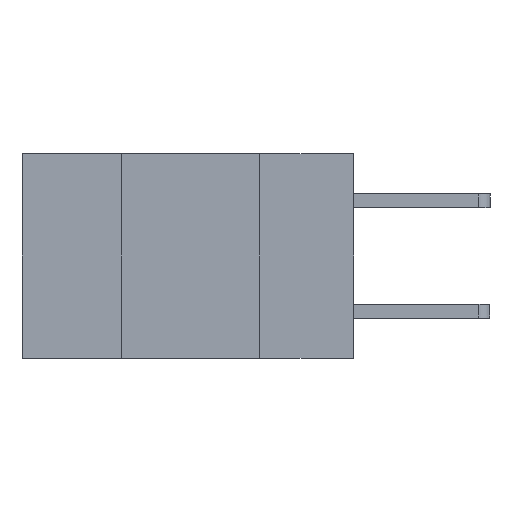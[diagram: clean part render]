
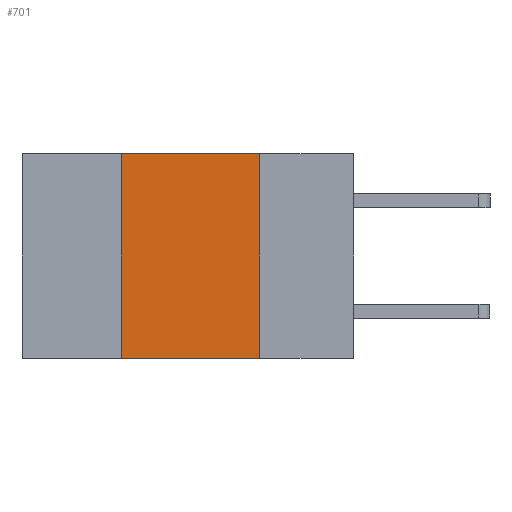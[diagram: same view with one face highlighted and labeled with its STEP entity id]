
A CAD part, left-side view. The second image highlights one B-rep face of the part: STEP entity #701.
In plain terms, the highlighted planar face has unit normal (-1, 0, 0).
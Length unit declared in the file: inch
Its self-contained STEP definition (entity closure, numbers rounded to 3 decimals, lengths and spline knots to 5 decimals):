
#74 = CARTESIAN_POINT ( 'NONE',  ( 0., 0.17, 0. ) ) ;
#165 = DIRECTION ( 'NONE',  ( 1., 0., 0. ) ) ;
#363 = ORIENTED_EDGE ( 'NONE', *, *, #1320, .T. ) ;
#701 = ADVANCED_FACE ( 'NONE', ( #8901 ), #9004, .F. ) ;
#724 = VERTEX_POINT ( 'NONE', #8096 ) ;
#1230 = CARTESIAN_POINT ( 'NONE',  ( 0., 0.42, -0.37 ) ) ;
#1320 = EDGE_CURVE ( 'NONE', #3982, #724, #2113, .T. ) ;
#1330 = DIRECTION ( 'NONE',  ( 0., -1., 0. ) ) ;
#1464 = CARTESIAN_POINT ( 'NONE',  ( 0., 0.17, 0. ) ) ;
#1579 = AXIS2_PLACEMENT_3D ( 'NONE', #6501, #165, #2660 ) ;
#1698 = VECTOR ( 'NONE', #4646, 39.37008 ) ;
#2113 = LINE ( 'NONE', #5324, #5716 ) ;
#2286 = VERTEX_POINT ( 'NONE', #1464 ) ;
#2660 = DIRECTION ( 'NONE',  ( 0., 0., -1. ) ) ;
#3022 = CARTESIAN_POINT ( 'NONE',  ( 0., 0.6, 0. ) ) ;
#3110 = EDGE_CURVE ( 'NONE', #9505, #2286, #3909, .T. ) ;
#3909 = LINE ( 'NONE', #3022, #8797 ) ;
#3982 = VERTEX_POINT ( 'NONE', #1230 ) ;
#4424 = CARTESIAN_POINT ( 'NONE',  ( 0., 0.42, 0. ) ) ;
#4646 = DIRECTION ( 'NONE',  ( 0., 0., 1. ) ) ;
#5324 = CARTESIAN_POINT ( 'NONE',  ( 0., 0.6, -0.37 ) ) ;
#5429 = LINE ( 'NONE', #74, #7710 ) ;
#5450 = CARTESIAN_POINT ( 'NONE',  ( 0., 0.42, 0. ) ) ;
#5674 = EDGE_LOOP ( 'NONE', ( #5904, #7659, #6311, #363 ) ) ;
#5716 = VECTOR ( 'NONE', #1330, 39.37008 ) ;
#5760 = EDGE_CURVE ( 'NONE', #3982, #9505, #6789, .T. ) ;
#5904 = ORIENTED_EDGE ( 'NONE', *, *, #5909, .F. ) ;
#5909 = EDGE_CURVE ( 'NONE', #2286, #724, #5429, .T. ) ;
#6311 = ORIENTED_EDGE ( 'NONE', *, *, #5760, .F. ) ;
#6501 = CARTESIAN_POINT ( 'NONE',  ( 0., 0.6, 0. ) ) ;
#6789 = LINE ( 'NONE', #4424, #1698 ) ;
#7659 = ORIENTED_EDGE ( 'NONE', *, *, #3110, .F. ) ;
#7710 = VECTOR ( 'NONE', #7905, 39.37008 ) ;
#7905 = DIRECTION ( 'NONE',  ( 0., 0., -1. ) ) ;
#8096 = CARTESIAN_POINT ( 'NONE',  ( 0., 0.17, -0.37 ) ) ;
#8797 = VECTOR ( 'NONE', #9356, 39.37008 ) ;
#8901 = FACE_OUTER_BOUND ( 'NONE', #5674, .T. ) ;
#9004 = PLANE ( 'NONE',  #1579 ) ;
#9356 = DIRECTION ( 'NONE',  ( 0., -1., 0. ) ) ;
#9505 = VERTEX_POINT ( 'NONE', #5450 ) ;
